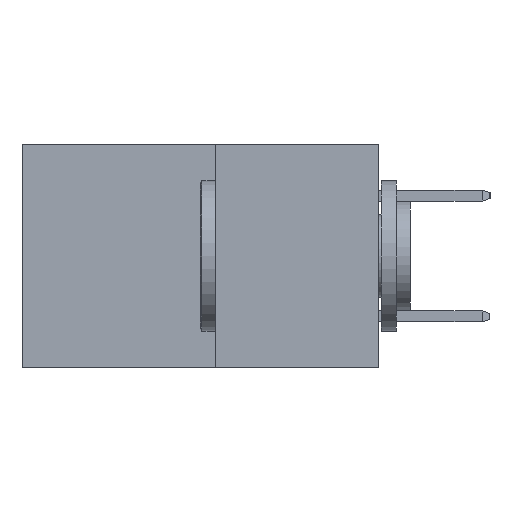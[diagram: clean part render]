
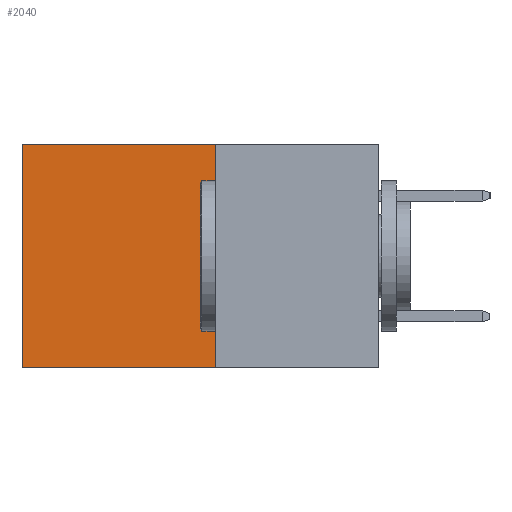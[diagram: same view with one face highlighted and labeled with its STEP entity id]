
A CAD part, left-side view. The second image highlights one B-rep face of the part: STEP entity #2040.
In plain terms, the highlighted planar face has unit normal (-1, 0, 0).
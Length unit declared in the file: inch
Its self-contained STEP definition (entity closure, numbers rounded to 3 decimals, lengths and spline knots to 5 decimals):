
#147 = CARTESIAN_POINT ( 'NONE',  ( 0.277, 0.27, -0.37 ) ) ;
#213 = VECTOR ( 'NONE', #8746, 39.37008 ) ;
#520 = CARTESIAN_POINT ( 'NONE',  ( 0.277, 0.59, -0.37 ) ) ;
#865 = DIRECTION ( 'NONE',  ( 0., 0., -1. ) ) ;
#869 = LINE ( 'NONE', #8831, #213 ) ;
#952 = PLANE ( 'NONE',  #11923 ) ;
#1123 = CARTESIAN_POINT ( 'NONE',  ( 0.277, 0.27, -0.37 ) ) ;
#1749 = EDGE_CURVE ( 'NONE', #12926, #11617, #6820, .T. ) ;
#1860 = VECTOR ( 'NONE', #5755, 39.37008 ) ;
#2040 = ADVANCED_FACE ( 'NONE', ( #3240 ), #952, .F. ) ;
#2207 = LINE ( 'NONE', #5918, #10076 ) ;
#2828 = DIRECTION ( 'NONE',  ( 0., 1., 0. ) ) ;
#3240 = FACE_OUTER_BOUND ( 'NONE', #12508, .T. ) ;
#3389 = VERTEX_POINT ( 'NONE', #5192 ) ;
#4541 = EDGE_CURVE ( 'NONE', #11617, #13180, #7400, .T. ) ;
#4652 = EDGE_CURVE ( 'NONE', #3389, #13180, #869, .T. ) ;
#5192 = CARTESIAN_POINT ( 'NONE',  ( 0.277, 0.59, 0. ) ) ;
#5620 = DIRECTION ( 'NONE',  ( 1., 0., 0. ) ) ;
#5755 = DIRECTION ( 'NONE',  ( 0., 1., 0. ) ) ;
#5834 = ORIENTED_EDGE ( 'NONE', *, *, #12651, .T. ) ;
#5918 = CARTESIAN_POINT ( 'NONE',  ( 0.277, 0.27, 0. ) ) ;
#6325 = CARTESIAN_POINT ( 'NONE',  ( 0.277, 0.27, 0. ) ) ;
#6502 = VECTOR ( 'NONE', #865, 39.37008 ) ;
#6706 = CARTESIAN_POINT ( 'NONE',  ( 0.277, 0.27, -0.37 ) ) ;
#6820 = LINE ( 'NONE', #1123, #6502 ) ;
#7354 = CARTESIAN_POINT ( 'NONE',  ( 0.277, 0.27, -0.37 ) ) ;
#7400 = LINE ( 'NONE', #6706, #1860 ) ;
#8248 = ORIENTED_EDGE ( 'NONE', *, *, #1749, .F. ) ;
#8746 = DIRECTION ( 'NONE',  ( 0., 0., -1. ) ) ;
#8831 = CARTESIAN_POINT ( 'NONE',  ( 0.277, 0.59, -0.37 ) ) ;
#8878 = ORIENTED_EDGE ( 'NONE', *, *, #4652, .T. ) ;
#10076 = VECTOR ( 'NONE', #2828, 39.37008 ) ;
#11563 = ORIENTED_EDGE ( 'NONE', *, *, #4541, .F. ) ;
#11617 = VERTEX_POINT ( 'NONE', #7354 ) ;
#11923 = AXIS2_PLACEMENT_3D ( 'NONE', #147, #5620, #12100 ) ;
#12100 = DIRECTION ( 'NONE',  ( 0., 0., -1. ) ) ;
#12508 = EDGE_LOOP ( 'NONE', ( #8878, #11563, #8248, #5834 ) ) ;
#12651 = EDGE_CURVE ( 'NONE', #12926, #3389, #2207, .T. ) ;
#12926 = VERTEX_POINT ( 'NONE', #6325 ) ;
#13180 = VERTEX_POINT ( 'NONE', #520 ) ;
